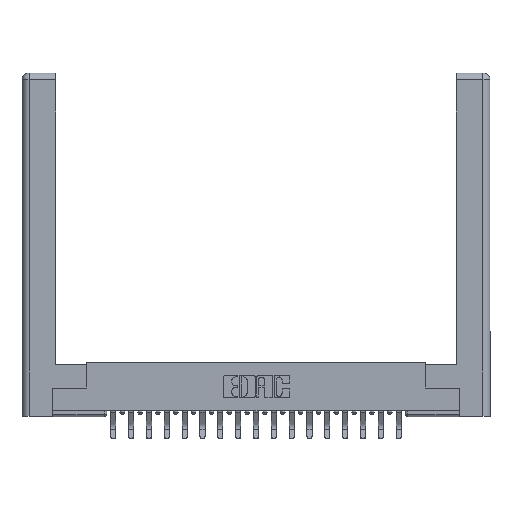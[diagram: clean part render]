
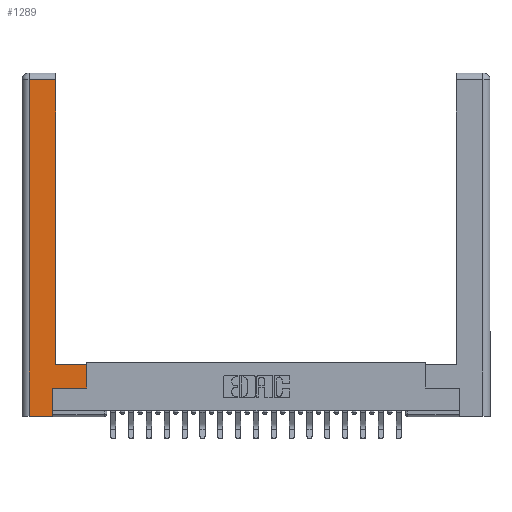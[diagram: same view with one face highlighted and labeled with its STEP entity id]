
A CAD part, top view. The second image highlights one B-rep face of the part: STEP entity #1289.
In plain terms, the highlighted planar face has unit normal (0, 0, 1).
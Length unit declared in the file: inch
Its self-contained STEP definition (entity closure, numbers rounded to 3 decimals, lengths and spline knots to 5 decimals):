
#669 = LINE ( 'NONE', #5110, #3710 ) ;
#716 = CARTESIAN_POINT ( 'NONE',  ( 0.565, 0.245, 0. ) ) ;
#1289 = ADVANCED_FACE ( 'NONE', ( #5083 ), #7671, .F. ) ;
#1380 = ORIENTED_EDGE ( 'NONE', *, *, #9533, .T. ) ;
#1568 = CARTESIAN_POINT ( 'NONE',  ( 0.565, 0.245, 0. ) ) ;
#1806 = CARTESIAN_POINT ( 'NONE',  ( 0.0615, 0., 0. ) ) ;
#1850 = DIRECTION ( 'NONE',  ( 0., 1., 0. ) ) ;
#1855 = ORIENTED_EDGE ( 'NONE', *, *, #5284, .T. ) ;
#1987 = EDGE_LOOP ( 'NONE', ( #13967, #5904, #1380, #11158, #2798, #14786, #1855, #16617 ) ) ;
#2187 = LINE ( 'NONE', #6290, #20163 ) ;
#2430 = AXIS2_PLACEMENT_3D ( 'NONE', #10812, #12515, #18965 ) ;
#2513 = LINE ( 'NONE', #18409, #18707 ) ;
#2798 = ORIENTED_EDGE ( 'NONE', *, *, #12736, .T. ) ;
#2874 = VECTOR ( 'NONE', #7938, 39.37008 ) ;
#3537 = VECTOR ( 'NONE', #4302, 39.37008 ) ;
#3710 = VECTOR ( 'NONE', #1850, 39.37008 ) ;
#3813 = LINE ( 'NONE', #1806, #12159 ) ;
#4302 = DIRECTION ( 'NONE',  ( 0., 1., 0. ) ) ;
#5083 = FACE_OUTER_BOUND ( 'NONE', #1987, .T. ) ;
#5110 = CARTESIAN_POINT ( 'NONE',  ( 0.295, 3., 0. ) ) ;
#5173 = CARTESIAN_POINT ( 'NONE',  ( 0.0615, 0., 0. ) ) ;
#5284 = EDGE_CURVE ( 'NONE', #18021, #5714, #20108, .T. ) ;
#5714 = VERTEX_POINT ( 'NONE', #7702 ) ;
#5864 = CARTESIAN_POINT ( 'NONE',  ( 0.265, 0.245, 0. ) ) ;
#5904 = ORIENTED_EDGE ( 'NONE', *, *, #6588, .T. ) ;
#6290 = CARTESIAN_POINT ( 'NONE',  ( 0.0615, 2.94, 0. ) ) ;
#6419 = CARTESIAN_POINT ( 'NONE',  ( 0.265, 0., 0. ) ) ;
#6588 = EDGE_CURVE ( 'NONE', #15721, #11261, #2187, .T. ) ;
#7671 = PLANE ( 'NONE',  #2430 ) ;
#7702 = CARTESIAN_POINT ( 'NONE',  ( 0.565, 0.45, 0. ) ) ;
#7938 = DIRECTION ( 'NONE',  ( 1., 0., 0. ) ) ;
#8728 = EDGE_CURVE ( 'NONE', #14598, #18021, #10424, .T. ) ;
#8867 = DIRECTION ( 'NONE',  ( -1., 0., 0. ) ) ;
#9431 = EDGE_CURVE ( 'NONE', #12468, #11144, #17243, .T. ) ;
#9533 = EDGE_CURVE ( 'NONE', #11261, #12468, #3813, .T. ) ;
#9643 = DIRECTION ( 'NONE',  ( 1., 0., 0. ) ) ;
#10424 = LINE ( 'NONE', #1568, #2874 ) ;
#10468 = VECTOR ( 'NONE', #12191, 39.37008 ) ;
#10534 = VERTEX_POINT ( 'NONE', #12929 ) ;
#10812 = CARTESIAN_POINT ( 'NONE',  ( 0., 0., 0. ) ) ;
#11144 = VERTEX_POINT ( 'NONE', #14477 ) ;
#11158 = ORIENTED_EDGE ( 'NONE', *, *, #9431, .T. ) ;
#11261 = VERTEX_POINT ( 'NONE', #12974 ) ;
#12159 = VECTOR ( 'NONE', #19752, 39.37008 ) ;
#12191 = DIRECTION ( 'NONE',  ( 0., 1., 0. ) ) ;
#12468 = VERTEX_POINT ( 'NONE', #5173 ) ;
#12515 = DIRECTION ( 'NONE',  ( 0., 0., -1. ) ) ;
#12736 = EDGE_CURVE ( 'NONE', #11144, #14598, #16731, .T. ) ;
#12929 = CARTESIAN_POINT ( 'NONE',  ( 0.295, 0.45, 0. ) ) ;
#12937 = VECTOR ( 'NONE', #9643, 39.37008 ) ;
#12974 = CARTESIAN_POINT ( 'NONE',  ( 0.0615, 2.94, 0. ) ) ;
#13425 = DIRECTION ( 'NONE',  ( -1., 0., 0. ) ) ;
#13820 = CARTESIAN_POINT ( 'NONE',  ( 0.565, 0.45, 0. ) ) ;
#13853 = EDGE_CURVE ( 'NONE', #5714, #10534, #2513, .T. ) ;
#13967 = ORIENTED_EDGE ( 'NONE', *, *, #20429, .T. ) ;
#14477 = CARTESIAN_POINT ( 'NONE',  ( 0.265, 0., 0. ) ) ;
#14598 = VERTEX_POINT ( 'NONE', #20025 ) ;
#14786 = ORIENTED_EDGE ( 'NONE', *, *, #8728, .T. ) ;
#15721 = VERTEX_POINT ( 'NONE', #19974 ) ;
#16617 = ORIENTED_EDGE ( 'NONE', *, *, #13853, .T. ) ;
#16731 = LINE ( 'NONE', #5864, #3537 ) ;
#17243 = LINE ( 'NONE', #6419, #12937 ) ;
#18021 = VERTEX_POINT ( 'NONE', #716 ) ;
#18409 = CARTESIAN_POINT ( 'NONE',  ( 0.295, 0.45, 0. ) ) ;
#18707 = VECTOR ( 'NONE', #8867, 39.37008 ) ;
#18965 = DIRECTION ( 'NONE',  ( -1., 0., 0. ) ) ;
#19752 = DIRECTION ( 'NONE',  ( 0., -1., 0. ) ) ;
#19974 = CARTESIAN_POINT ( 'NONE',  ( 0.295, 2.94, 0. ) ) ;
#20025 = CARTESIAN_POINT ( 'NONE',  ( 0.265, 0.245, 0. ) ) ;
#20108 = LINE ( 'NONE', #13820, #10468 ) ;
#20163 = VECTOR ( 'NONE', #13425, 39.37008 ) ;
#20429 = EDGE_CURVE ( 'NONE', #10534, #15721, #669, .T. ) ;
